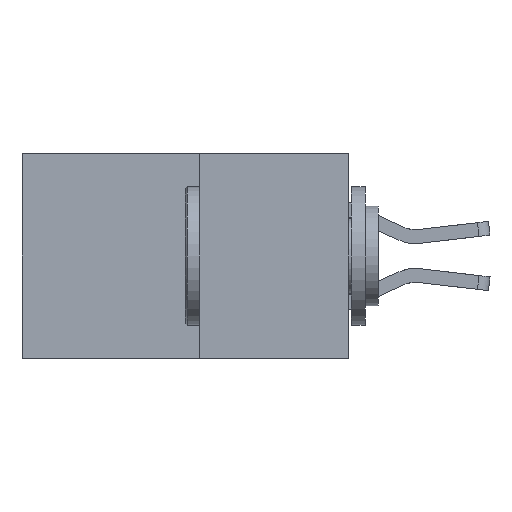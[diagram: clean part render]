
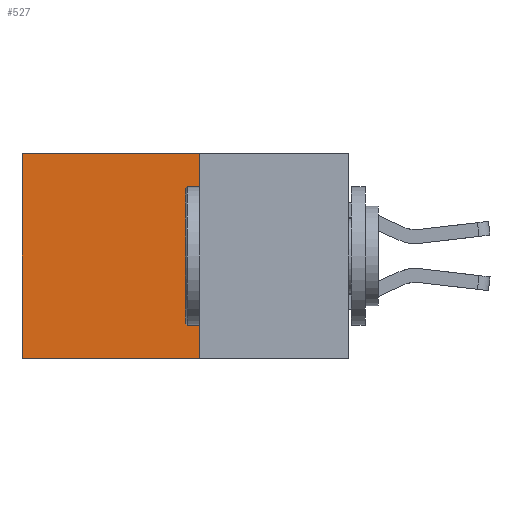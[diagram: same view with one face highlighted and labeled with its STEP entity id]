
A CAD part, left-side view. The second image highlights one B-rep face of the part: STEP entity #527.
In plain terms, the highlighted planar face has unit normal (-1, 0, 0).
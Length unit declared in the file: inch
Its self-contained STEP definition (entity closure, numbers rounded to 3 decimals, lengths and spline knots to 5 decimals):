
#139 = ORIENTED_EDGE ( 'NONE', *, *, #4219, .F. ) ;
#527 = ADVANCED_FACE ( 'NONE', ( #8902 ), #3255, .F. ) ;
#595 = EDGE_LOOP ( 'NONE', ( #6765, #5257, #139, #4484 ) ) ;
#709 = LINE ( 'NONE', #7196, #4361 ) ;
#1163 = DIRECTION ( 'NONE',  ( 0., 1., 0. ) ) ;
#1227 = VERTEX_POINT ( 'NONE', #4105 ) ;
#1383 = VECTOR ( 'NONE', #8949, 39.37008 ) ;
#1609 = LINE ( 'NONE', #3896, #1383 ) ;
#1734 = CARTESIAN_POINT ( 'NONE',  ( 0.277, 0.59, -0.37 ) ) ;
#1748 = VERTEX_POINT ( 'NONE', #3522 ) ;
#3255 = PLANE ( 'NONE',  #6047 ) ;
#3362 = EDGE_CURVE ( 'NONE', #1227, #1748, #709, .T. ) ;
#3522 = CARTESIAN_POINT ( 'NONE',  ( 0.277, 0.59, -0.37 ) ) ;
#3896 = CARTESIAN_POINT ( 'NONE',  ( 0.277, 0.27, -0.37 ) ) ;
#3927 = CARTESIAN_POINT ( 'NONE',  ( 0.277, 0.59, 0. ) ) ;
#4105 = CARTESIAN_POINT ( 'NONE',  ( 0.277, 0.27, -0.37 ) ) ;
#4219 = EDGE_CURVE ( 'NONE', #6677, #1227, #1609, .T. ) ;
#4232 = EDGE_CURVE ( 'NONE', #4243, #1748, #8854, .T. ) ;
#4243 = VERTEX_POINT ( 'NONE', #3927 ) ;
#4361 = VECTOR ( 'NONE', #1163, 39.37008 ) ;
#4442 = LINE ( 'NONE', #6750, #7818 ) ;
#4484 = ORIENTED_EDGE ( 'NONE', *, *, #5476, .T. ) ;
#4618 = DIRECTION ( 'NONE',  ( 0., 1., 0. ) ) ;
#4620 = CARTESIAN_POINT ( 'NONE',  ( 0.277, 0.27, -0.37 ) ) ;
#5257 = ORIENTED_EDGE ( 'NONE', *, *, #3362, .F. ) ;
#5384 = DIRECTION ( 'NONE',  ( 0., 0., -1. ) ) ;
#5423 = DIRECTION ( 'NONE',  ( 1., 0., 0. ) ) ;
#5476 = EDGE_CURVE ( 'NONE', #6677, #4243, #4442, .T. ) ;
#5905 = CARTESIAN_POINT ( 'NONE',  ( 0.277, 0.27, 0. ) ) ;
#6047 = AXIS2_PLACEMENT_3D ( 'NONE', #4620, #5423, #5384 ) ;
#6677 = VERTEX_POINT ( 'NONE', #5905 ) ;
#6715 = VECTOR ( 'NONE', #8224, 39.37008 ) ;
#6750 = CARTESIAN_POINT ( 'NONE',  ( 0.277, 0.27, 0. ) ) ;
#6765 = ORIENTED_EDGE ( 'NONE', *, *, #4232, .T. ) ;
#7196 = CARTESIAN_POINT ( 'NONE',  ( 0.277, 0.27, -0.37 ) ) ;
#7818 = VECTOR ( 'NONE', #4618, 39.37008 ) ;
#8224 = DIRECTION ( 'NONE',  ( 0., 0., -1. ) ) ;
#8854 = LINE ( 'NONE', #1734, #6715 ) ;
#8902 = FACE_OUTER_BOUND ( 'NONE', #595, .T. ) ;
#8949 = DIRECTION ( 'NONE',  ( 0., 0., -1. ) ) ;
